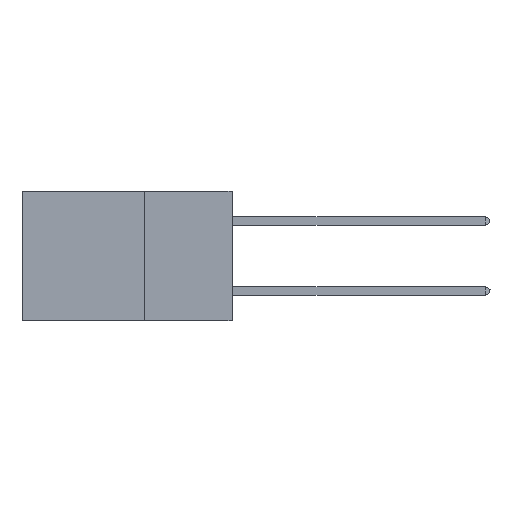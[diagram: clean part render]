
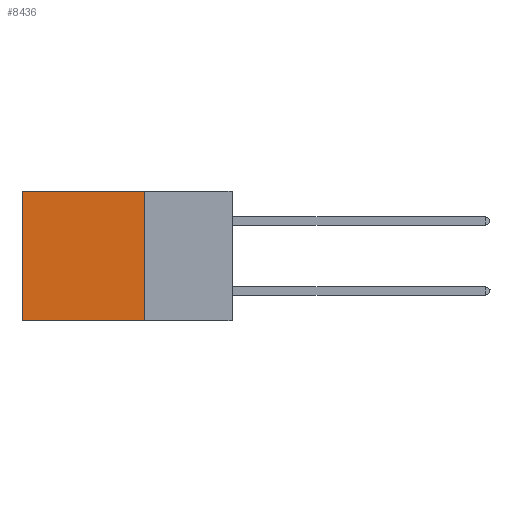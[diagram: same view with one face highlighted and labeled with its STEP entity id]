
A CAD part, left-side view. The second image highlights one B-rep face of the part: STEP entity #8436.
In plain terms, the highlighted planar face has unit normal (-1, 0, 0).
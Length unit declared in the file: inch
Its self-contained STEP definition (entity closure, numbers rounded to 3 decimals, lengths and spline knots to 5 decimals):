
#1607 = CARTESIAN_POINT ( 'NONE',  ( 0.2875, 0.25, 0. ) ) ;
#2073 = VECTOR ( 'NONE', #3957, 39.37008 ) ;
#2252 = VECTOR ( 'NONE', #15904, 39.37008 ) ;
#3688 = CARTESIAN_POINT ( 'NONE',  ( 0.2875, 0.6, 0. ) ) ;
#3957 = DIRECTION ( 'NONE',  ( 0., 0., -1. ) ) ;
#4555 = DIRECTION ( 'NONE',  ( 0., 0., -1. ) ) ;
#5456 = PLANE ( 'NONE',  #10050 ) ;
#5766 = VERTEX_POINT ( 'NONE', #14007 ) ;
#7442 = LINE ( 'NONE', #10933, #9875 ) ;
#7813 = CARTESIAN_POINT ( 'NONE',  ( 0.2875, 0.25, 0. ) ) ;
#8436 = ADVANCED_FACE ( 'NONE', ( #12658 ), #5456, .F. ) ;
#8938 = LINE ( 'NONE', #13439, #2252 ) ;
#9875 = VECTOR ( 'NONE', #4555, 39.37008 ) ;
#10050 = AXIS2_PLACEMENT_3D ( 'NONE', #7813, #16634, #12202 ) ;
#10933 = CARTESIAN_POINT ( 'NONE',  ( 0.2875, 0.25, 0. ) ) ;
#11755 = VERTEX_POINT ( 'NONE', #12889 ) ;
#12202 = DIRECTION ( 'NONE',  ( 0., 0., -1. ) ) ;
#12658 = FACE_OUTER_BOUND ( 'NONE', #28274, .T. ) ;
#12659 = EDGE_CURVE ( 'NONE', #11755, #20043, #8938, .T. ) ;
#12889 = CARTESIAN_POINT ( 'NONE',  ( 0.2875, 0.25, -0.37 ) ) ;
#13313 = ORIENTED_EDGE ( 'NONE', *, *, #20414, .F. ) ;
#13439 = CARTESIAN_POINT ( 'NONE',  ( 0.2875, 0.25, -0.37 ) ) ;
#13692 = ORIENTED_EDGE ( 'NONE', *, *, #12659, .F. ) ;
#14007 = CARTESIAN_POINT ( 'NONE',  ( 0.2875, 0.25, 0. ) ) ;
#15030 = CARTESIAN_POINT ( 'NONE',  ( 0.2875, 0.6, 0. ) ) ;
#15749 = VERTEX_POINT ( 'NONE', #3688 ) ;
#15904 = DIRECTION ( 'NONE',  ( 0., 1., 0. ) ) ;
#16308 = EDGE_CURVE ( 'NONE', #15749, #20043, #23853, .T. ) ;
#16634 = DIRECTION ( 'NONE',  ( 1., 0., 0. ) ) ;
#18055 = VECTOR ( 'NONE', #28707, 39.37008 ) ;
#18439 = EDGE_CURVE ( 'NONE', #5766, #15749, #27242, .T. ) ;
#19069 = ORIENTED_EDGE ( 'NONE', *, *, #18439, .T. ) ;
#20043 = VERTEX_POINT ( 'NONE', #23410 ) ;
#20414 = EDGE_CURVE ( 'NONE', #5766, #11755, #7442, .T. ) ;
#23410 = CARTESIAN_POINT ( 'NONE',  ( 0.2875, 0.6, -0.37 ) ) ;
#23853 = LINE ( 'NONE', #15030, #2073 ) ;
#27242 = LINE ( 'NONE', #1607, #18055 ) ;
#27323 = ORIENTED_EDGE ( 'NONE', *, *, #16308, .T. ) ;
#28274 = EDGE_LOOP ( 'NONE', ( #27323, #13692, #13313, #19069 ) ) ;
#28707 = DIRECTION ( 'NONE',  ( 0., 1., 0. ) ) ;
